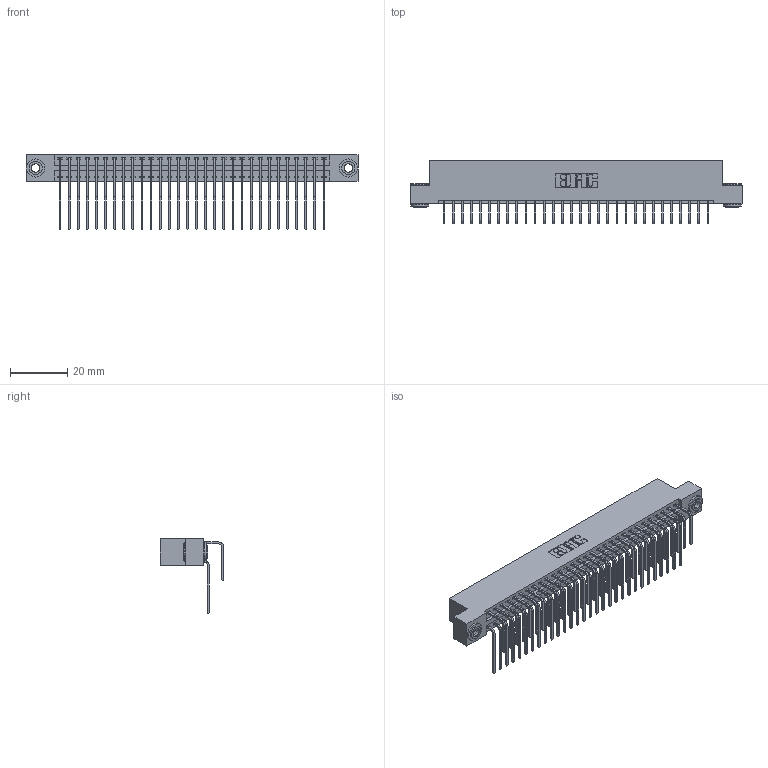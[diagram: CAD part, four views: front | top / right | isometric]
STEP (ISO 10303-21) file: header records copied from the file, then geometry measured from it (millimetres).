
FILE_DESCRIPTION (( 'STEP AP203' ), '1' );
FILE_NAME ('346-060-558-203.STEP', '2018-08-28T06:16:17', ( '' ), ( '' ), 'SwSTEP 2.0', 'SolidWorks 2016', '' );
FILE_SCHEMA (( 'CONFIG_CONTROL_DESIGN' ));
Length unit declared in the file: inch
Products named in the file (5): 345-292-001_558 Tail - 2; 345-250-002_345-250-002-102; 346-060-558-203; 346 Part_Flush Mounting Lugs - 0.156 Dia-TH; 345-292-001_558 559 Tail - 1
Assembly tree (63 placements, depth 2):
  346-060-558-203
    346 Part_Flush Mounting Lugs - 0.156 Dia-TH
    345-292-001_558 559 Tail - 1  x30
    345-292-001_558 Tail - 2  x30
    345-250-002_345-250-002-102  x2
Bounding box: 115.82 x 22.16 x 26.16 mm (x, y, z)
Volume: 11566.6 mm3; surface area: 17585.1 mm2
Topology: 63 solids, 63 shells, 3400 faces, 10065 edges, 6626 vertices
Faces by surface type: plane 2306, cylinder 1086, cone 8
Entity records: 23628 total; most frequent: CARTESIAN_POINT 3938, ORIENTED_EDGE 3814, DIRECTION 3525, EDGE_CURVE 1907, LINE 1591, VECTOR 1591, VERTEX_POINT 1266, AXIS2_PLACEMENT_3D 967
